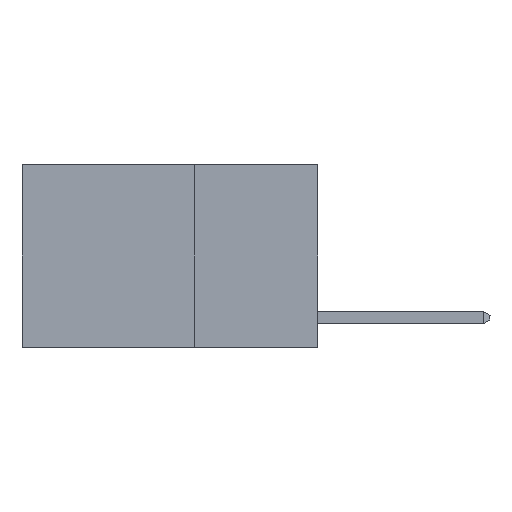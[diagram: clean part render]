
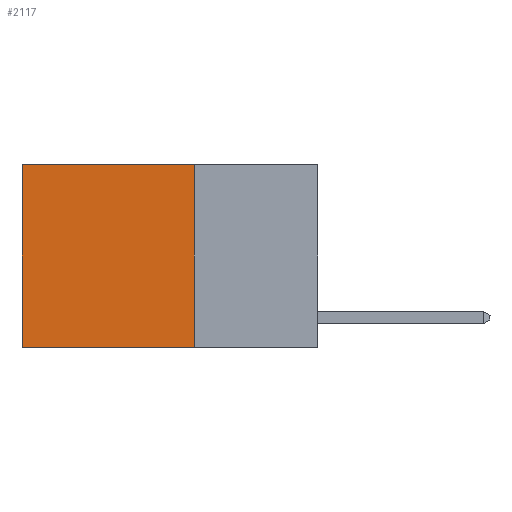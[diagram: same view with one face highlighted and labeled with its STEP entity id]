
A CAD part, left-side view. The second image highlights one B-rep face of the part: STEP entity #2117.
In plain terms, the highlighted planar face has unit normal (-1, 0, 0).
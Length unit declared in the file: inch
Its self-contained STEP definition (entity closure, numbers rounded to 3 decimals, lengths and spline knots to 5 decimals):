
#1281 = VECTOR ( 'NONE', #4316, 39.37008 ) ;
#1340 = CARTESIAN_POINT ( 'NONE',  ( 0.2625, 0.6, 0. ) ) ;
#1761 = CARTESIAN_POINT ( 'NONE',  ( 0.2625, 0.25, 0. ) ) ;
#2117 = ADVANCED_FACE ( 'NONE', ( #17952 ), #5077, .F. ) ;
#2145 = DIRECTION ( 'NONE',  ( 1., 0., 0. ) ) ;
#2412 = EDGE_LOOP ( 'NONE', ( #3372, #2531, #2423, #10144 ) ) ;
#2423 = ORIENTED_EDGE ( 'NONE', *, *, #4846, .F. ) ;
#2531 = ORIENTED_EDGE ( 'NONE', *, *, #3095, .F. ) ;
#3095 = EDGE_CURVE ( 'NONE', #8224, #13922, #3579, .T. ) ;
#3292 = DIRECTION ( 'NONE',  ( 0., 0., -1. ) ) ;
#3372 = ORIENTED_EDGE ( 'NONE', *, *, #18391, .T. ) ;
#3579 = LINE ( 'NONE', #8384, #8917 ) ;
#4316 = DIRECTION ( 'NONE',  ( 0., 0., -1. ) ) ;
#4846 = EDGE_CURVE ( 'NONE', #14032, #8224, #6588, .T. ) ;
#4992 = LINE ( 'NONE', #12852, #19442 ) ;
#5077 = PLANE ( 'NONE',  #20079 ) ;
#5823 = DIRECTION ( 'NONE',  ( 0., 1., 0. ) ) ;
#6588 = LINE ( 'NONE', #7241, #1281 ) ;
#7241 = CARTESIAN_POINT ( 'NONE',  ( 0.2625, 0.25, 0. ) ) ;
#7598 = LINE ( 'NONE', #15453, #7645 ) ;
#7645 = VECTOR ( 'NONE', #5823, 39.37008 ) ;
#8224 = VERTEX_POINT ( 'NONE', #9101 ) ;
#8384 = CARTESIAN_POINT ( 'NONE',  ( 0.2625, 0.25, -0.37 ) ) ;
#8917 = VECTOR ( 'NONE', #13010, 39.37008 ) ;
#9101 = CARTESIAN_POINT ( 'NONE',  ( 0.2625, 0.25, -0.37 ) ) ;
#9707 = CARTESIAN_POINT ( 'NONE',  ( 0.2625, 0.6, -0.37 ) ) ;
#10144 = ORIENTED_EDGE ( 'NONE', *, *, #14277, .T. ) ;
#12852 = CARTESIAN_POINT ( 'NONE',  ( 0.2625, 0.6, 0. ) ) ;
#13010 = DIRECTION ( 'NONE',  ( 0., 1., 0. ) ) ;
#13043 = CARTESIAN_POINT ( 'NONE',  ( 0.2625, 0.25, 0. ) ) ;
#13922 = VERTEX_POINT ( 'NONE', #9707 ) ;
#14032 = VERTEX_POINT ( 'NONE', #1761 ) ;
#14277 = EDGE_CURVE ( 'NONE', #14032, #18273, #7598, .T. ) ;
#15453 = CARTESIAN_POINT ( 'NONE',  ( 0.2625, 0.25, 0. ) ) ;
#17450 = DIRECTION ( 'NONE',  ( 0., 0., -1. ) ) ;
#17952 = FACE_OUTER_BOUND ( 'NONE', #2412, .T. ) ;
#18273 = VERTEX_POINT ( 'NONE', #1340 ) ;
#18391 = EDGE_CURVE ( 'NONE', #18273, #13922, #4992, .T. ) ;
#19442 = VECTOR ( 'NONE', #17450, 39.37008 ) ;
#20079 = AXIS2_PLACEMENT_3D ( 'NONE', #13043, #2145, #3292 ) ;
